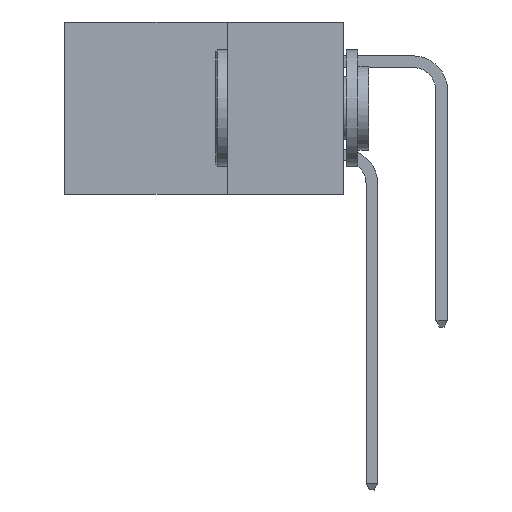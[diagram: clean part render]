
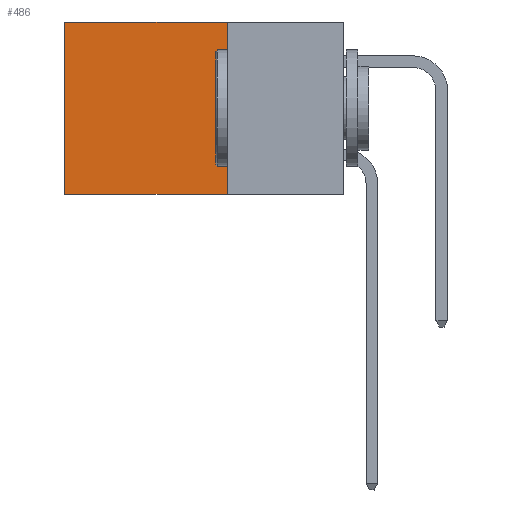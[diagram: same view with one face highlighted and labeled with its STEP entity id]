
A CAD part, left-side view. The second image highlights one B-rep face of the part: STEP entity #486.
In plain terms, the highlighted planar face has unit normal (-1, 0, 0).
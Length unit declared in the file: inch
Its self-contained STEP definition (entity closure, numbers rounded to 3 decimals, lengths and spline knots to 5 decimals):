
#27 = CARTESIAN_POINT ( 'NONE',  ( 0.2615, 0.6, -0.37 ) ) ;
#486 = ADVANCED_FACE ( 'NONE', ( #12736 ), #14787, .F. ) ;
#491 = CARTESIAN_POINT ( 'NONE',  ( 0.2615, 0.25, -0.37 ) ) ;
#525 = DIRECTION ( 'NONE',  ( 0., 1., 0. ) ) ;
#1116 = AXIS2_PLACEMENT_3D ( 'NONE', #19695, #9713, #14680 ) ;
#2072 = DIRECTION ( 'NONE',  ( 0., 0., -1. ) ) ;
#4112 = ORIENTED_EDGE ( 'NONE', *, *, #13599, .F. ) ;
#4604 = VERTEX_POINT ( 'NONE', #21069 ) ;
#4794 = VECTOR ( 'NONE', #2072, 39.37008 ) ;
#4998 = DIRECTION ( 'NONE',  ( 0., 1., 0. ) ) ;
#5375 = DIRECTION ( 'NONE',  ( 0., 0., -1. ) ) ;
#5384 = EDGE_CURVE ( 'NONE', #9949, #15833, #10897, .T. ) ;
#5975 = EDGE_LOOP ( 'NONE', ( #10134, #14724, #4112, #16139 ) ) ;
#7328 = CARTESIAN_POINT ( 'NONE',  ( 0.2615, 0.6, -0.37 ) ) ;
#8207 = LINE ( 'NONE', #14823, #10422 ) ;
#9713 = DIRECTION ( 'NONE',  ( 1., 0., 0. ) ) ;
#9949 = VERTEX_POINT ( 'NONE', #17612 ) ;
#10119 = VECTOR ( 'NONE', #5375, 39.37008 ) ;
#10134 = ORIENTED_EDGE ( 'NONE', *, *, #19279, .T. ) ;
#10277 = VECTOR ( 'NONE', #525, 39.37008 ) ;
#10422 = VECTOR ( 'NONE', #4998, 39.37008 ) ;
#10897 = LINE ( 'NONE', #15650, #10277 ) ;
#11846 = EDGE_CURVE ( 'NONE', #19273, #4604, #8207, .T. ) ;
#12213 = LINE ( 'NONE', #7328, #4794 ) ;
#12263 = LINE ( 'NONE', #491, #10119 ) ;
#12736 = FACE_OUTER_BOUND ( 'NONE', #5975, .T. ) ;
#13599 = EDGE_CURVE ( 'NONE', #19273, #9949, #12263, .T. ) ;
#14680 = DIRECTION ( 'NONE',  ( 0., 0., -1. ) ) ;
#14724 = ORIENTED_EDGE ( 'NONE', *, *, #5384, .F. ) ;
#14787 = PLANE ( 'NONE',  #1116 ) ;
#14823 = CARTESIAN_POINT ( 'NONE',  ( 0.2615, 0.25, 0. ) ) ;
#15650 = CARTESIAN_POINT ( 'NONE',  ( 0.2615, 0.25, -0.37 ) ) ;
#15833 = VERTEX_POINT ( 'NONE', #27 ) ;
#16139 = ORIENTED_EDGE ( 'NONE', *, *, #11846, .T. ) ;
#16857 = CARTESIAN_POINT ( 'NONE',  ( 0.2615, 0.25, 0. ) ) ;
#17612 = CARTESIAN_POINT ( 'NONE',  ( 0.2615, 0.25, -0.37 ) ) ;
#19273 = VERTEX_POINT ( 'NONE', #16857 ) ;
#19279 = EDGE_CURVE ( 'NONE', #4604, #15833, #12213, .T. ) ;
#19695 = CARTESIAN_POINT ( 'NONE',  ( 0.2615, 0.25, -0.37 ) ) ;
#21069 = CARTESIAN_POINT ( 'NONE',  ( 0.2615, 0.6, 0. ) ) ;
